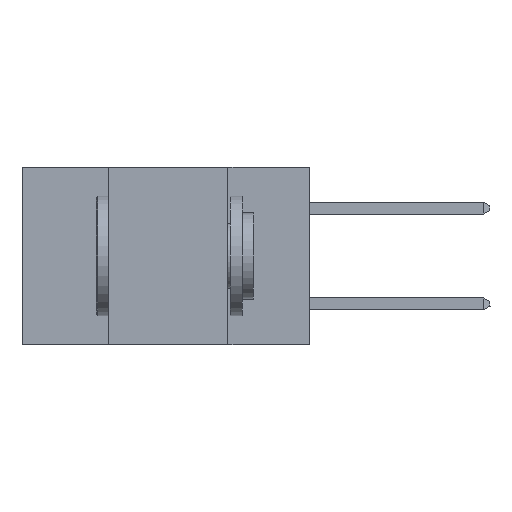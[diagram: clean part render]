
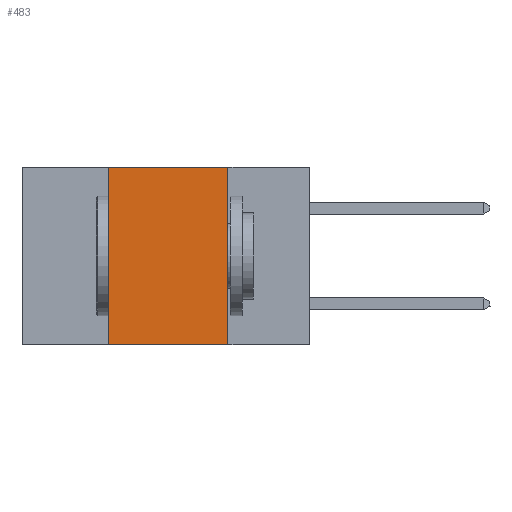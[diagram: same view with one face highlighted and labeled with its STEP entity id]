
A CAD part, left-side view. The second image highlights one B-rep face of the part: STEP entity #483.
In plain terms, the highlighted planar face has unit normal (-1, 0, 0).
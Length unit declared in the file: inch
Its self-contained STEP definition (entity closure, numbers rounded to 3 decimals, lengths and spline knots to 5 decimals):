
#353 = VERTEX_POINT ( 'NONE', #564 ) ;
#482 = VECTOR ( 'NONE', #2165, 39.37008 ) ;
#483 = ADVANCED_FACE ( 'NONE', ( #5283 ), #832, .F. ) ;
#564 = CARTESIAN_POINT ( 'NONE',  ( 0., 0.17, -0.37 ) ) ;
#778 = LINE ( 'NONE', #11053, #482 ) ;
#832 = PLANE ( 'NONE',  #7763 ) ;
#1386 = EDGE_LOOP ( 'NONE', ( #8637, #2243, #3433, #3715 ) ) ;
#1783 = VERTEX_POINT ( 'NONE', #7188 ) ;
#2021 = EDGE_CURVE ( 'NONE', #2368, #4292, #4130, .T. ) ;
#2165 = DIRECTION ( 'NONE',  ( 0., -1., 0. ) ) ;
#2243 = ORIENTED_EDGE ( 'NONE', *, *, #8015, .F. ) ;
#2368 = VERTEX_POINT ( 'NONE', #2921 ) ;
#2484 = EDGE_CURVE ( 'NONE', #2368, #353, #11172, .T. ) ;
#2921 = CARTESIAN_POINT ( 'NONE',  ( 0., 0.42, -0.37 ) ) ;
#3433 = ORIENTED_EDGE ( 'NONE', *, *, #2021, .F. ) ;
#3715 = ORIENTED_EDGE ( 'NONE', *, *, #2484, .T. ) ;
#4130 = LINE ( 'NONE', #6625, #4698 ) ;
#4292 = VERTEX_POINT ( 'NONE', #7105 ) ;
#4668 = EDGE_CURVE ( 'NONE', #1783, #353, #6907, .T. ) ;
#4698 = VECTOR ( 'NONE', #6819, 39.37008 ) ;
#4822 = CARTESIAN_POINT ( 'NONE',  ( 0., 0.6, 0. ) ) ;
#5072 = CARTESIAN_POINT ( 'NONE',  ( 0., 0.17, 0. ) ) ;
#5236 = DIRECTION ( 'NONE',  ( 0., 0., -1. ) ) ;
#5283 = FACE_OUTER_BOUND ( 'NONE', #1386, .T. ) ;
#6529 = DIRECTION ( 'NONE',  ( 1., 0., 0. ) ) ;
#6615 = VECTOR ( 'NONE', #5236, 39.37008 ) ;
#6625 = CARTESIAN_POINT ( 'NONE',  ( 0., 0.42, 0. ) ) ;
#6819 = DIRECTION ( 'NONE',  ( 0., 0., 1. ) ) ;
#6907 = LINE ( 'NONE', #5072, #6615 ) ;
#7105 = CARTESIAN_POINT ( 'NONE',  ( 0., 0.42, 0. ) ) ;
#7188 = CARTESIAN_POINT ( 'NONE',  ( 0., 0.17, 0. ) ) ;
#7763 = AXIS2_PLACEMENT_3D ( 'NONE', #4822, #6529, #10632 ) ;
#8015 = EDGE_CURVE ( 'NONE', #4292, #1783, #778, .T. ) ;
#8637 = ORIENTED_EDGE ( 'NONE', *, *, #4668, .F. ) ;
#8897 = VECTOR ( 'NONE', #10806, 39.37008 ) ;
#10632 = DIRECTION ( 'NONE',  ( 0., 0., -1. ) ) ;
#10806 = DIRECTION ( 'NONE',  ( 0., -1., 0. ) ) ;
#11053 = CARTESIAN_POINT ( 'NONE',  ( 0., 0.6, 0. ) ) ;
#11172 = LINE ( 'NONE', #11497, #8897 ) ;
#11497 = CARTESIAN_POINT ( 'NONE',  ( 0., 0.6, -0.37 ) ) ;
